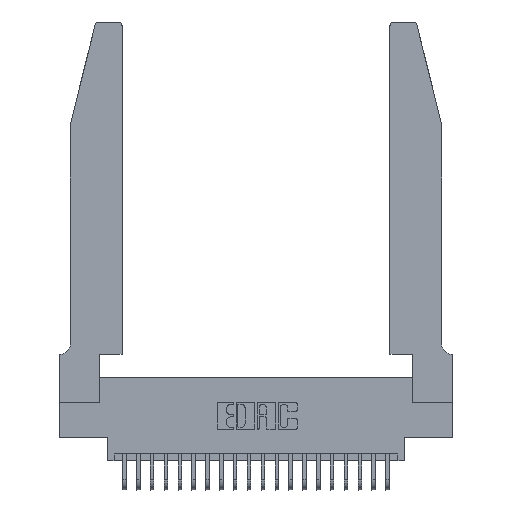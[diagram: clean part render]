
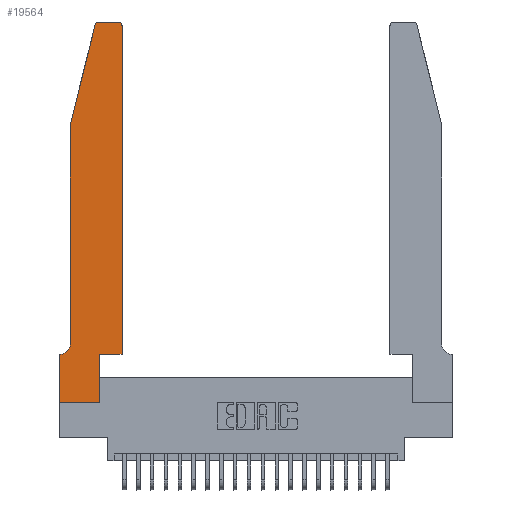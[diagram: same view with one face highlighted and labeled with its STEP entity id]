
A CAD part, top view. The second image highlights one B-rep face of the part: STEP entity #19564.
In plain terms, the highlighted planar face has unit normal (0, 0, 1).
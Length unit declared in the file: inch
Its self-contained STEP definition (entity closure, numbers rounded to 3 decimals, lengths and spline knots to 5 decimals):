
#106 = AXIS2_PLACEMENT_3D ( 'NONE', #21170, #19299, #17051 ) ;
#211 = VERTEX_POINT ( 'NONE', #22323 ) ;
#221 = VECTOR ( 'NONE', #2548, 39.37008 ) ;
#283 = ORIENTED_EDGE ( 'NONE', *, *, #7107, .T. ) ;
#392 = DIRECTION ( 'NONE',  ( -1., 0., 0. ) ) ;
#412 = EDGE_CURVE ( 'NONE', #7956, #23782, #13599, .T. ) ;
#691 = VECTOR ( 'NONE', #10184, 39.37008 ) ;
#1119 = EDGE_CURVE ( 'NONE', #3057, #211, #19693, .T. ) ;
#1677 = CARTESIAN_POINT ( 'NONE',  ( 0.4205, 2.75, 0.37 ) ) ;
#2016 = VECTOR ( 'NONE', #5786, 39.37008 ) ;
#2024 = EDGE_CURVE ( 'NONE', #17951, #5819, #12651, .T. ) ;
#2538 = VECTOR ( 'NONE', #3525, 39.37008 ) ;
#2548 = DIRECTION ( 'NONE',  ( -1., 0., 0. ) ) ;
#2697 = CARTESIAN_POINT ( 'NONE',  ( 0.25487, 2.72718, 0.37 ) ) ;
#2773 = CIRCLE ( 'NONE', #7483, 0.03 ) ;
#3057 = VERTEX_POINT ( 'NONE', #13543 ) ;
#3525 = DIRECTION ( 'NONE',  ( 0., 1., 0. ) ) ;
#4375 = VERTEX_POINT ( 'NONE', #17477 ) ;
#4379 = ORIENTED_EDGE ( 'NONE', *, *, #19258, .T. ) ;
#4941 = CARTESIAN_POINT ( 'NONE',  ( 0.4205, 2.72, 0.37 ) ) ;
#5239 = CARTESIAN_POINT ( 'NONE',  ( 0., 0., 0.37 ) ) ;
#5432 = EDGE_CURVE ( 'NONE', #5819, #5764, #14776, .T. ) ;
#5748 = CARTESIAN_POINT ( 'NONE',  ( 0.4505, 0.35, 0.37 ) ) ;
#5764 = VERTEX_POINT ( 'NONE', #13985 ) ;
#5786 = DIRECTION ( 'NONE',  ( 0., -1., 0. ) ) ;
#5819 = VERTEX_POINT ( 'NONE', #10729 ) ;
#5901 = AXIS2_PLACEMENT_3D ( 'NONE', #4941, #18545, #10704 ) ;
#6282 = ORIENTED_EDGE ( 'NONE', *, *, #1119, .T. ) ;
#6327 = CARTESIAN_POINT ( 'NONE',  ( 0.284, 2.72, 0.37 ) ) ;
#6387 = CARTESIAN_POINT ( 'NONE',  ( 0.0755, 2., 0.37 ) ) ;
#6472 = DIRECTION ( 'NONE',  ( 0., 0., 1. ) ) ;
#6659 = CIRCLE ( 'NONE', #5901, 0.03 ) ;
#6683 = VECTOR ( 'NONE', #13816, 39.37008 ) ;
#6899 = ORIENTED_EDGE ( 'NONE', *, *, #13838, .T. ) ;
#6991 = AXIS2_PLACEMENT_3D ( 'NONE', #17311, #13567, #392 ) ;
#7107 = EDGE_CURVE ( 'NONE', #8772, #13927, #7677, .T. ) ;
#7483 = AXIS2_PLACEMENT_3D ( 'NONE', #6327, #6472, #18991 ) ;
#7677 = LINE ( 'NONE', #9349, #2538 ) ;
#7956 = VERTEX_POINT ( 'NONE', #1677 ) ;
#8413 = ORIENTED_EDGE ( 'NONE', *, *, #19420, .T. ) ;
#8772 = VERTEX_POINT ( 'NONE', #10478 ) ;
#9172 = ORIENTED_EDGE ( 'NONE', *, *, #14636, .T. ) ;
#9349 = CARTESIAN_POINT ( 'NONE',  ( 0.4505, 0.35, 0.37 ) ) ;
#10184 = DIRECTION ( 'NONE',  ( 0., -1., 0. ) ) ;
#10213 = DIRECTION ( 'NONE',  ( -0.239, -0.971, 0. ) ) ;
#10478 = CARTESIAN_POINT ( 'NONE',  ( 0.4505, 0.35, 0.37 ) ) ;
#10704 = DIRECTION ( 'NONE',  ( 1., 0., 0. ) ) ;
#10729 = CARTESIAN_POINT ( 'NONE',  ( 0., 0.35, 0.37 ) ) ;
#10784 = CARTESIAN_POINT ( 'NONE',  ( 0.4505, 2.72, 0.37 ) ) ;
#11267 = LINE ( 'NONE', #6387, #19209 ) ;
#12219 = CARTESIAN_POINT ( 'NONE',  ( 0.2605, 2.75, 0.37 ) ) ;
#12651 = LINE ( 'NONE', #19708, #15390 ) ;
#12690 = EDGE_CURVE ( 'NONE', #17588, #4375, #15604, .T. ) ;
#13440 = ORIENTED_EDGE ( 'NONE', *, *, #5432, .T. ) ;
#13543 = CARTESIAN_POINT ( 'NONE',  ( 0.2865, 0., 0.37 ) ) ;
#13567 = DIRECTION ( 'NONE',  ( 0., 0., -1. ) ) ;
#13599 = LINE ( 'NONE', #12219, #221 ) ;
#13816 = DIRECTION ( 'NONE',  ( 1., 0., 0. ) ) ;
#13838 = EDGE_CURVE ( 'NONE', #4375, #17951, #19828, .T. ) ;
#13927 = VERTEX_POINT ( 'NONE', #10784 ) ;
#13985 = CARTESIAN_POINT ( 'NONE',  ( 0., 0., 0.37 ) ) ;
#14500 = EDGE_CURVE ( 'NONE', #23613, #17588, #11267, .T. ) ;
#14606 = ORIENTED_EDGE ( 'NONE', *, *, #412, .T. ) ;
#14617 = LINE ( 'NONE', #5748, #6683 ) ;
#14636 = EDGE_CURVE ( 'NONE', #23782, #23613, #2773, .T. ) ;
#14776 = LINE ( 'NONE', #15488, #2016 ) ;
#14778 = VECTOR ( 'NONE', #20184, 39.37008 ) ;
#15054 = EDGE_CURVE ( 'NONE', #13927, #7956, #6659, .T. ) ;
#15180 = CARTESIAN_POINT ( 'NONE',  ( 0.0055, 0.35, 0.37 ) ) ;
#15390 = VECTOR ( 'NONE', #15912, 39.37008 ) ;
#15488 = CARTESIAN_POINT ( 'NONE',  ( 0., 0., 0.37 ) ) ;
#15604 = LINE ( 'NONE', #21881, #691 ) ;
#15912 = DIRECTION ( 'NONE',  ( -1., 0., 0. ) ) ;
#17051 = DIRECTION ( 'NONE',  ( 1., 0., 0. ) ) ;
#17311 = CARTESIAN_POINT ( 'NONE',  ( 0.0055, 0.42, 0.37 ) ) ;
#17477 = CARTESIAN_POINT ( 'NONE',  ( 0.0755, 0.42, 0.37 ) ) ;
#17588 = VERTEX_POINT ( 'NONE', #23656 ) ;
#17951 = VERTEX_POINT ( 'NONE', #15180 ) ;
#18545 = DIRECTION ( 'NONE',  ( 0., 0., 1. ) ) ;
#18991 = DIRECTION ( 'NONE',  ( 1., 0., 0. ) ) ;
#19132 = PLANE ( 'NONE',  #106 ) ;
#19209 = VECTOR ( 'NONE', #10213, 39.37008 ) ;
#19258 = EDGE_CURVE ( 'NONE', #5764, #3057, #25034, .T. ) ;
#19299 = DIRECTION ( 'NONE',  ( 0., 0., 1. ) ) ;
#19407 = CARTESIAN_POINT ( 'NONE',  ( 0.284, 2.75, 0.37 ) ) ;
#19420 = EDGE_CURVE ( 'NONE', #211, #8772, #14617, .T. ) ;
#19564 = ADVANCED_FACE ( 'NONE', ( #23163 ), #19132, .T. ) ;
#19693 = LINE ( 'NONE', #23851, #14778 ) ;
#19708 = CARTESIAN_POINT ( 'NONE',  ( 0.0755, 0.35, 0.37 ) ) ;
#19828 = CIRCLE ( 'NONE', #6991, 0.07 ) ;
#20184 = DIRECTION ( 'NONE',  ( 0., 1., 0. ) ) ;
#20295 = ORIENTED_EDGE ( 'NONE', *, *, #2024, .T. ) ;
#20733 = VECTOR ( 'NONE', #24925, 39.37008 ) ;
#20926 = EDGE_LOOP ( 'NONE', ( #14606, #9172, #24370, #23880, #6899, #20295, #13440, #4379, #6282, #8413, #283, #24708 ) ) ;
#21170 = CARTESIAN_POINT ( 'NONE',  ( 0., 0.35, 0.37 ) ) ;
#21881 = CARTESIAN_POINT ( 'NONE',  ( 0.0755, 2., 0.37 ) ) ;
#22323 = CARTESIAN_POINT ( 'NONE',  ( 0.2865, 0.35, 0.37 ) ) ;
#23163 = FACE_OUTER_BOUND ( 'NONE', #20926, .T. ) ;
#23613 = VERTEX_POINT ( 'NONE', #2697 ) ;
#23656 = CARTESIAN_POINT ( 'NONE',  ( 0.0755, 2., 0.37 ) ) ;
#23782 = VERTEX_POINT ( 'NONE', #19407 ) ;
#23851 = CARTESIAN_POINT ( 'NONE',  ( 0.2865, 0.35, 0.37 ) ) ;
#23880 = ORIENTED_EDGE ( 'NONE', *, *, #12690, .T. ) ;
#24370 = ORIENTED_EDGE ( 'NONE', *, *, #14500, .T. ) ;
#24708 = ORIENTED_EDGE ( 'NONE', *, *, #15054, .T. ) ;
#24925 = DIRECTION ( 'NONE',  ( 1., 0., 0. ) ) ;
#25034 = LINE ( 'NONE', #5239, #20733 ) ;
